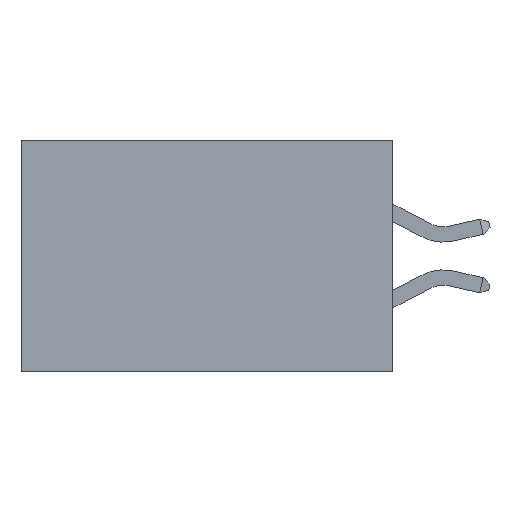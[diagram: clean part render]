
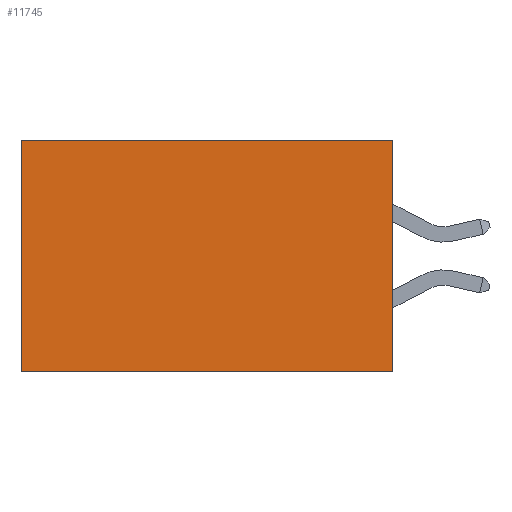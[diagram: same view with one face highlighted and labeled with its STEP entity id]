
A CAD part, left-side view. The second image highlights one B-rep face of the part: STEP entity #11745.
In plain terms, the highlighted planar face has unit normal (-1, 0, 0).
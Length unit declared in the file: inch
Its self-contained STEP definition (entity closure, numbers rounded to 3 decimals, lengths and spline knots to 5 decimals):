
#468 = CARTESIAN_POINT ( 'NONE',  ( 0.2875, 0., 0. ) ) ;
#734 = DIRECTION ( 'NONE',  ( 1., 0., 0. ) ) ;
#842 = CARTESIAN_POINT ( 'NONE',  ( 0.2875, 0., 0. ) ) ;
#1005 = LINE ( 'NONE', #12457, #5581 ) ;
#1774 = CARTESIAN_POINT ( 'NONE',  ( 0.2875, 0., -0.375 ) ) ;
#1784 = CARTESIAN_POINT ( 'NONE',  ( 0.2875, 0.6, -0.375 ) ) ;
#1792 = EDGE_CURVE ( 'NONE', #4686, #12704, #2498, .T. ) ;
#2498 = LINE ( 'NONE', #6699, #4949 ) ;
#3182 = VECTOR ( 'NONE', #11535, 39.37008 ) ;
#3695 = VECTOR ( 'NONE', #11101, 39.37008 ) ;
#4686 = VERTEX_POINT ( 'NONE', #468 ) ;
#4817 = EDGE_CURVE ( 'NONE', #6922, #10484, #5773, .T. ) ;
#4949 = VECTOR ( 'NONE', #11678, 39.37008 ) ;
#5581 = VECTOR ( 'NONE', #6312, 39.37008 ) ;
#5668 = EDGE_CURVE ( 'NONE', #4686, #6922, #7117, .T. ) ;
#5773 = LINE ( 'NONE', #1784, #3695 ) ;
#6160 = EDGE_CURVE ( 'NONE', #12704, #10484, #1005, .T. ) ;
#6312 = DIRECTION ( 'NONE',  ( 0., 1., 0. ) ) ;
#6352 = CARTESIAN_POINT ( 'NONE',  ( 0.2875, 0.6, -0.375 ) ) ;
#6699 = CARTESIAN_POINT ( 'NONE',  ( 0.2875, 0., -0.375 ) ) ;
#6922 = VERTEX_POINT ( 'NONE', #6977 ) ;
#6977 = CARTESIAN_POINT ( 'NONE',  ( 0.2875, 0.6, 0. ) ) ;
#7000 = PLANE ( 'NONE',  #13621 ) ;
#7117 = LINE ( 'NONE', #842, #3182 ) ;
#7712 = ORIENTED_EDGE ( 'NONE', *, *, #6160, .F. ) ;
#10484 = VERTEX_POINT ( 'NONE', #6352 ) ;
#11101 = DIRECTION ( 'NONE',  ( 0., 0., -1. ) ) ;
#11535 = DIRECTION ( 'NONE',  ( 0., 1., 0. ) ) ;
#11624 = ORIENTED_EDGE ( 'NONE', *, *, #5668, .T. ) ;
#11678 = DIRECTION ( 'NONE',  ( 0., 0., -1. ) ) ;
#11745 = ADVANCED_FACE ( 'NONE', ( #12177 ), #7000, .F. ) ;
#12177 = FACE_OUTER_BOUND ( 'NONE', #13441, .T. ) ;
#12221 = ORIENTED_EDGE ( 'NONE', *, *, #1792, .F. ) ;
#12313 = DIRECTION ( 'NONE',  ( 0., 0., -1. ) ) ;
#12457 = CARTESIAN_POINT ( 'NONE',  ( 0.2875, 0., -0.375 ) ) ;
#12553 = CARTESIAN_POINT ( 'NONE',  ( 0.2875, 0., -0.375 ) ) ;
#12704 = VERTEX_POINT ( 'NONE', #12553 ) ;
#13424 = ORIENTED_EDGE ( 'NONE', *, *, #4817, .T. ) ;
#13441 = EDGE_LOOP ( 'NONE', ( #13424, #7712, #12221, #11624 ) ) ;
#13621 = AXIS2_PLACEMENT_3D ( 'NONE', #1774, #734, #12313 ) ;
